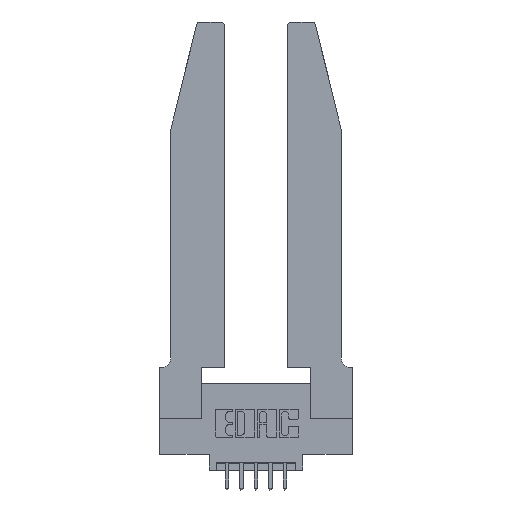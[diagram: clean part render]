
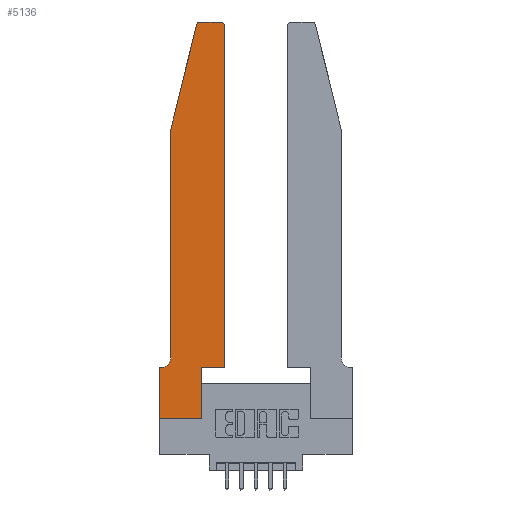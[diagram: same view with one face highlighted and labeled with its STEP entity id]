
A CAD part, top view. The second image highlights one B-rep face of the part: STEP entity #5136.
In plain terms, the highlighted planar face has unit normal (0, 0, 1).
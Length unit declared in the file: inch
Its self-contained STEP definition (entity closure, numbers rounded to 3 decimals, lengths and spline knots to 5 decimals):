
#143 = CARTESIAN_POINT ( 'NONE',  ( 0.0755, 0.35, 0.37 ) ) ;
#417 = LINE ( 'NONE', #1656, #11500 ) ;
#453 = ORIENTED_EDGE ( 'NONE', *, *, #12379, .T. ) ;
#562 = EDGE_CURVE ( 'NONE', #4705, #3615, #1734, .T. ) ;
#848 = LINE ( 'NONE', #10614, #7568 ) ;
#1057 = VECTOR ( 'NONE', #11060, 39.37008 ) ;
#1386 = DIRECTION ( 'NONE',  ( 1., 0., 0. ) ) ;
#1413 = LINE ( 'NONE', #1420, #1057 ) ;
#1420 = CARTESIAN_POINT ( 'NONE',  ( 0.0755, 2., 0.37 ) ) ;
#1509 = CARTESIAN_POINT ( 'NONE',  ( 0.4205, 2.72, 0.37 ) ) ;
#1528 = CARTESIAN_POINT ( 'NONE',  ( 0.4505, 2.72, 0.37 ) ) ;
#1569 = DIRECTION ( 'NONE',  ( 0., 0., 1. ) ) ;
#1656 = CARTESIAN_POINT ( 'NONE',  ( 0., 0., 0.37 ) ) ;
#1734 = CIRCLE ( 'NONE', #5016, 0.03 ) ;
#1829 = ORIENTED_EDGE ( 'NONE', *, *, #8493, .T. ) ;
#1831 = VECTOR ( 'NONE', #5738, 39.37008 ) ;
#1865 = VECTOR ( 'NONE', #5454, 39.37008 ) ;
#1898 = EDGE_CURVE ( 'NONE', #6520, #4705, #13144, .T. ) ;
#2026 = EDGE_CURVE ( 'NONE', #3615, #2237, #11538, .T. ) ;
#2059 = CARTESIAN_POINT ( 'NONE',  ( 0.0755, 2., 0.37 ) ) ;
#2237 = VERTEX_POINT ( 'NONE', #8181 ) ;
#2339 = EDGE_LOOP ( 'NONE', ( #7020, #12479, #6667, #10749, #453, #1829, #12539, #10312, #3169, #2519, #5965, #5964 ) ) ;
#2469 = CARTESIAN_POINT ( 'NONE',  ( 0.25487, 2.72718, 0.37 ) ) ;
#2507 = EDGE_CURVE ( 'NONE', #2237, #9666, #12168, .T. ) ;
#2519 = ORIENTED_EDGE ( 'NONE', *, *, #10703, .T. ) ;
#2848 = CARTESIAN_POINT ( 'NONE',  ( 0.4505, 0.35, 0.37 ) ) ;
#3161 = DIRECTION ( 'NONE',  ( 0., 1., 0. ) ) ;
#3167 = VECTOR ( 'NONE', #12750, 39.37008 ) ;
#3169 = ORIENTED_EDGE ( 'NONE', *, *, #12206, .T. ) ;
#3540 = VERTEX_POINT ( 'NONE', #10041 ) ;
#3615 = VERTEX_POINT ( 'NONE', #9562 ) ;
#4027 = VERTEX_POINT ( 'NONE', #11753 ) ;
#4367 = EDGE_CURVE ( 'NONE', #9971, #6519, #417, .T. ) ;
#4616 = DIRECTION ( 'NONE',  ( -1., 0., 0. ) ) ;
#4665 = CARTESIAN_POINT ( 'NONE',  ( 0.2605, 2.75, 0.37 ) ) ;
#4705 = VERTEX_POINT ( 'NONE', #1528 ) ;
#4924 = VERTEX_POINT ( 'NONE', #9527 ) ;
#5016 = AXIS2_PLACEMENT_3D ( 'NONE', #1509, #12263, #10771 ) ;
#5127 = LINE ( 'NONE', #6646, #12765 ) ;
#5136 = ADVANCED_FACE ( 'NONE', ( #11003 ), #12176, .T. ) ;
#5143 = LINE ( 'NONE', #143, #1831 ) ;
#5454 = DIRECTION ( 'NONE',  ( 0., 1., 0. ) ) ;
#5482 = CARTESIAN_POINT ( 'NONE',  ( 0.4505, 0.35, 0.37 ) ) ;
#5738 = DIRECTION ( 'NONE',  ( -1., 0., 0. ) ) ;
#5964 = ORIENTED_EDGE ( 'NONE', *, *, #562, .T. ) ;
#5965 = ORIENTED_EDGE ( 'NONE', *, *, #1898, .T. ) ;
#6001 = DIRECTION ( 'NONE',  ( 0., 0., -1. ) ) ;
#6286 = AXIS2_PLACEMENT_3D ( 'NONE', #12200, #6001, #13235 ) ;
#6519 = VERTEX_POINT ( 'NONE', #9307 ) ;
#6520 = VERTEX_POINT ( 'NONE', #2848 ) ;
#6646 = CARTESIAN_POINT ( 'NONE',  ( 0., 0., 0.37 ) ) ;
#6667 = ORIENTED_EDGE ( 'NONE', *, *, #13324, .T. ) ;
#6675 = VERTEX_POINT ( 'NONE', #9485 ) ;
#6943 = EDGE_CURVE ( 'NONE', #4027, #3540, #1413, .T. ) ;
#7020 = ORIENTED_EDGE ( 'NONE', *, *, #2026, .T. ) ;
#7041 = AXIS2_PLACEMENT_3D ( 'NONE', #7279, #7483, #7533 ) ;
#7279 = CARTESIAN_POINT ( 'NONE',  ( 0.284, 2.72, 0.37 ) ) ;
#7483 = DIRECTION ( 'NONE',  ( 0., 0., 1. ) ) ;
#7498 = CARTESIAN_POINT ( 'NONE',  ( 0., 0., 0.37 ) ) ;
#7533 = DIRECTION ( 'NONE',  ( 1., 0., 0. ) ) ;
#7568 = VECTOR ( 'NONE', #3161, 39.37008 ) ;
#7908 = VERTEX_POINT ( 'NONE', #11327 ) ;
#8119 = CARTESIAN_POINT ( 'NONE',  ( 0., 0.35, 0.37 ) ) ;
#8181 = CARTESIAN_POINT ( 'NONE',  ( 0.284, 2.75, 0.37 ) ) ;
#8493 = EDGE_CURVE ( 'NONE', #7908, #4924, #5143, .T. ) ;
#8680 = VECTOR ( 'NONE', #9607, 39.37008 ) ;
#8837 = VECTOR ( 'NONE', #4616, 39.37008 ) ;
#9033 = EDGE_CURVE ( 'NONE', #4924, #9971, #5127, .T. ) ;
#9154 = DIRECTION ( 'NONE',  ( 1., 0., 0. ) ) ;
#9307 = CARTESIAN_POINT ( 'NONE',  ( 0.2865, 0., 0.37 ) ) ;
#9485 = CARTESIAN_POINT ( 'NONE',  ( 0.2865, 0.35, 0.37 ) ) ;
#9527 = CARTESIAN_POINT ( 'NONE',  ( 0., 0.35, 0.37 ) ) ;
#9562 = CARTESIAN_POINT ( 'NONE',  ( 0.4205, 2.75, 0.37 ) ) ;
#9607 = DIRECTION ( 'NONE',  ( -0.239, -0.971, 0. ) ) ;
#9666 = VERTEX_POINT ( 'NONE', #2469 ) ;
#9971 = VERTEX_POINT ( 'NONE', #7498 ) ;
#10041 = CARTESIAN_POINT ( 'NONE',  ( 0.0755, 0.42, 0.37 ) ) ;
#10312 = ORIENTED_EDGE ( 'NONE', *, *, #4367, .T. ) ;
#10614 = CARTESIAN_POINT ( 'NONE',  ( 0.2865, 0.35, 0.37 ) ) ;
#10703 = EDGE_CURVE ( 'NONE', #6675, #6520, #11927, .T. ) ;
#10749 = ORIENTED_EDGE ( 'NONE', *, *, #6943, .T. ) ;
#10771 = DIRECTION ( 'NONE',  ( 1., 0., 0. ) ) ;
#11003 = FACE_OUTER_BOUND ( 'NONE', #2339, .T. ) ;
#11060 = DIRECTION ( 'NONE',  ( 0., -1., 0. ) ) ;
#11327 = CARTESIAN_POINT ( 'NONE',  ( 0.0055, 0.35, 0.37 ) ) ;
#11500 = VECTOR ( 'NONE', #1386, 39.37008 ) ;
#11538 = LINE ( 'NONE', #4665, #8837 ) ;
#11753 = CARTESIAN_POINT ( 'NONE',  ( 0.0755, 2., 0.37 ) ) ;
#11770 = CARTESIAN_POINT ( 'NONE',  ( 0.4505, 0.35, 0.37 ) ) ;
#11927 = LINE ( 'NONE', #11770, #3167 ) ;
#12168 = CIRCLE ( 'NONE', #7041, 0.03 ) ;
#12176 = PLANE ( 'NONE',  #13249 ) ;
#12200 = CARTESIAN_POINT ( 'NONE',  ( 0.0055, 0.42, 0.37 ) ) ;
#12206 = EDGE_CURVE ( 'NONE', #6519, #6675, #848, .T. ) ;
#12263 = DIRECTION ( 'NONE',  ( 0., 0., 1. ) ) ;
#12379 = EDGE_CURVE ( 'NONE', #3540, #7908, #13483, .T. ) ;
#12479 = ORIENTED_EDGE ( 'NONE', *, *, #2507, .T. ) ;
#12539 = ORIENTED_EDGE ( 'NONE', *, *, #9033, .T. ) ;
#12750 = DIRECTION ( 'NONE',  ( 1., 0., 0. ) ) ;
#12765 = VECTOR ( 'NONE', #13824, 39.37008 ) ;
#13144 = LINE ( 'NONE', #5482, #1865 ) ;
#13235 = DIRECTION ( 'NONE',  ( -1., 0., 0. ) ) ;
#13249 = AXIS2_PLACEMENT_3D ( 'NONE', #8119, #1569, #9154 ) ;
#13324 = EDGE_CURVE ( 'NONE', #9666, #4027, #13774, .T. ) ;
#13483 = CIRCLE ( 'NONE', #6286, 0.07 ) ;
#13774 = LINE ( 'NONE', #2059, #8680 ) ;
#13824 = DIRECTION ( 'NONE',  ( 0., -1., 0. ) ) ;
